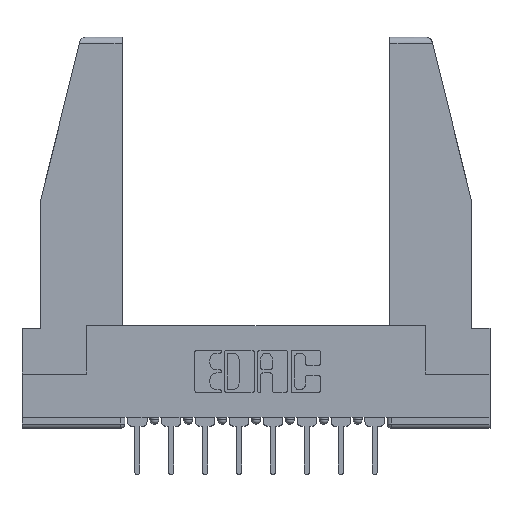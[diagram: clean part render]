
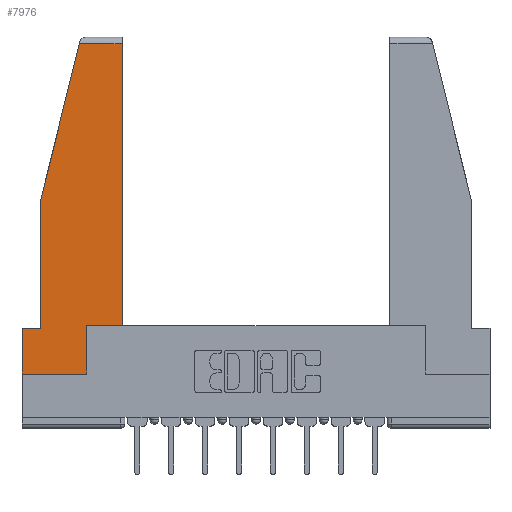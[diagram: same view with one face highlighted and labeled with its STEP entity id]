
A CAD part, top view. The second image highlights one B-rep face of the part: STEP entity #7976.
In plain terms, the highlighted planar face has unit normal (0, 0, 1).
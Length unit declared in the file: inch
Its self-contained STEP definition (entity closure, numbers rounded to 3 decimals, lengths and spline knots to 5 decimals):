
#333 = VECTOR ( 'NONE', #11538, 39.37008 ) ;
#337 = CARTESIAN_POINT ( 'NONE',  ( 0., 0.21, 0. ) ) ;
#397 = CARTESIAN_POINT ( 'NONE',  ( 0.271, 1.55, 0. ) ) ;
#437 = EDGE_CURVE ( 'NONE', #4911, #10769, #7629, .T. ) ;
#815 = DIRECTION ( 'NONE',  ( 0., 1., 0. ) ) ;
#1083 = LINE ( 'NONE', #10318, #12042 ) ;
#1299 = DIRECTION ( 'NONE',  ( 0., -1., 0. ) ) ;
#1390 = AXIS2_PLACEMENT_3D ( 'NONE', #6643, #8769, #13017 ) ;
#1481 = DIRECTION ( 'NONE',  ( -0.239, -0.971, 0. ) ) ;
#1785 = VERTEX_POINT ( 'NONE', #13434 ) ;
#1841 = ORIENTED_EDGE ( 'NONE', *, *, #8040, .T. ) ;
#2047 = VECTOR ( 'NONE', #6535, 39.37008 ) ;
#2300 = DIRECTION ( 'NONE',  ( 1., 0., 0. ) ) ;
#2301 = VECTOR ( 'NONE', #7746, 39.37008 ) ;
#2319 = CARTESIAN_POINT ( 'NONE',  ( 0.086, 0.8, 0. ) ) ;
#2370 = PLANE ( 'NONE',  #1390 ) ;
#2706 = LINE ( 'NONE', #6446, #2047 ) ;
#2876 = ORIENTED_EDGE ( 'NONE', *, *, #5052, .T. ) ;
#2981 = LINE ( 'NONE', #3497, #2301 ) ;
#3023 = VECTOR ( 'NONE', #8249, 39.37008 ) ;
#3315 = VERTEX_POINT ( 'NONE', #6708 ) ;
#3398 = EDGE_CURVE ( 'NONE', #8681, #12346, #2981, .T. ) ;
#3485 = CARTESIAN_POINT ( 'NONE',  ( 0.461, 0.223, 0. ) ) ;
#3497 = CARTESIAN_POINT ( 'NONE',  ( 0., 0.21, 0. ) ) ;
#3697 = FACE_OUTER_BOUND ( 'NONE', #6474, .T. ) ;
#4670 = CARTESIAN_POINT ( 'NONE',  ( 0.297, 0., 0. ) ) ;
#4741 = LINE ( 'NONE', #9628, #12687 ) ;
#4911 = VERTEX_POINT ( 'NONE', #9040 ) ;
#5052 = EDGE_CURVE ( 'NONE', #10769, #1785, #1083, .T. ) ;
#5499 = LINE ( 'NONE', #6138, #3023 ) ;
#6138 = CARTESIAN_POINT ( 'NONE',  ( 0., 0.21, 0. ) ) ;
#6446 = CARTESIAN_POINT ( 'NONE',  ( 0., 1.52, 0. ) ) ;
#6474 = EDGE_LOOP ( 'NONE', ( #2876, #1841, #9001, #13485, #8741, #11358, #11105, #9126, #8494 ) ) ;
#6517 = VECTOR ( 'NONE', #1299, 39.37008 ) ;
#6535 = DIRECTION ( 'NONE',  ( -1., 0., 0. ) ) ;
#6643 = CARTESIAN_POINT ( 'NONE',  ( 0., 0., 0. ) ) ;
#6708 = CARTESIAN_POINT ( 'NONE',  ( 0., 0., 0. ) ) ;
#7629 = LINE ( 'NONE', #8391, #333 ) ;
#7746 = DIRECTION ( 'NONE',  ( -1., 0., 0. ) ) ;
#7880 = CARTESIAN_POINT ( 'NONE',  ( 0.297, 0., 0. ) ) ;
#7969 = EDGE_CURVE ( 'NONE', #12679, #8681, #10988, .T. ) ;
#7976 = ADVANCED_FACE ( 'NONE', ( #3697 ), #2370, .T. ) ;
#8040 = EDGE_CURVE ( 'NONE', #1785, #10478, #2706, .T. ) ;
#8162 = CARTESIAN_POINT ( 'NONE',  ( 0.086, 0.8, 0. ) ) ;
#8249 = DIRECTION ( 'NONE',  ( 0., -1., 0. ) ) ;
#8391 = CARTESIAN_POINT ( 'NONE',  ( 0.297, 0.223, 0. ) ) ;
#8494 = ORIENTED_EDGE ( 'NONE', *, *, #437, .T. ) ;
#8681 = VERTEX_POINT ( 'NONE', #9469 ) ;
#8741 = ORIENTED_EDGE ( 'NONE', *, *, #3398, .T. ) ;
#8769 = DIRECTION ( 'NONE',  ( 0., 0., 1. ) ) ;
#8874 = EDGE_CURVE ( 'NONE', #8921, #4911, #12642, .T. ) ;
#8921 = VERTEX_POINT ( 'NONE', #4670 ) ;
#9001 = ORIENTED_EDGE ( 'NONE', *, *, #11658, .T. ) ;
#9040 = CARTESIAN_POINT ( 'NONE',  ( 0.297, 0.223, 0. ) ) ;
#9126 = ORIENTED_EDGE ( 'NONE', *, *, #8874, .T. ) ;
#9238 = EDGE_CURVE ( 'NONE', #12346, #3315, #5499, .T. ) ;
#9469 = CARTESIAN_POINT ( 'NONE',  ( 0.086, 0.21, 0. ) ) ;
#9628 = CARTESIAN_POINT ( 'NONE',  ( 0., 0., 0. ) ) ;
#9833 = VECTOR ( 'NONE', #10972, 39.37008 ) ;
#9895 = VECTOR ( 'NONE', #1481, 39.37008 ) ;
#10318 = CARTESIAN_POINT ( 'NONE',  ( 0.461, 0.223, 0. ) ) ;
#10478 = VERTEX_POINT ( 'NONE', #13450 ) ;
#10769 = VERTEX_POINT ( 'NONE', #3485 ) ;
#10972 = DIRECTION ( 'NONE',  ( 0., 1., 0. ) ) ;
#10988 = LINE ( 'NONE', #2319, #6517 ) ;
#11105 = ORIENTED_EDGE ( 'NONE', *, *, #12165, .T. ) ;
#11358 = ORIENTED_EDGE ( 'NONE', *, *, #9238, .T. ) ;
#11538 = DIRECTION ( 'NONE',  ( 1., 0., 0. ) ) ;
#11658 = EDGE_CURVE ( 'NONE', #10478, #12679, #13377, .T. ) ;
#12042 = VECTOR ( 'NONE', #815, 39.37008 ) ;
#12165 = EDGE_CURVE ( 'NONE', #3315, #8921, #4741, .T. ) ;
#12346 = VERTEX_POINT ( 'NONE', #337 ) ;
#12642 = LINE ( 'NONE', #7880, #9833 ) ;
#12679 = VERTEX_POINT ( 'NONE', #8162 ) ;
#12687 = VECTOR ( 'NONE', #2300, 39.37008 ) ;
#13017 = DIRECTION ( 'NONE',  ( 1., 0., 0. ) ) ;
#13377 = LINE ( 'NONE', #397, #9895 ) ;
#13434 = CARTESIAN_POINT ( 'NONE',  ( 0.461, 1.52, 0. ) ) ;
#13450 = CARTESIAN_POINT ( 'NONE',  ( 0.2636, 1.52, 0. ) ) ;
#13485 = ORIENTED_EDGE ( 'NONE', *, *, #7969, .T. ) ;
